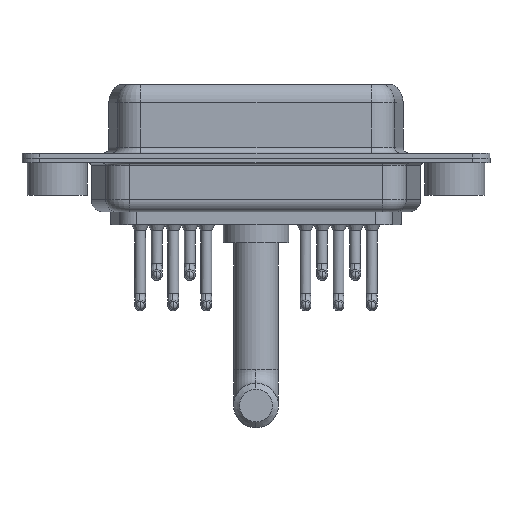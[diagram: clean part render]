
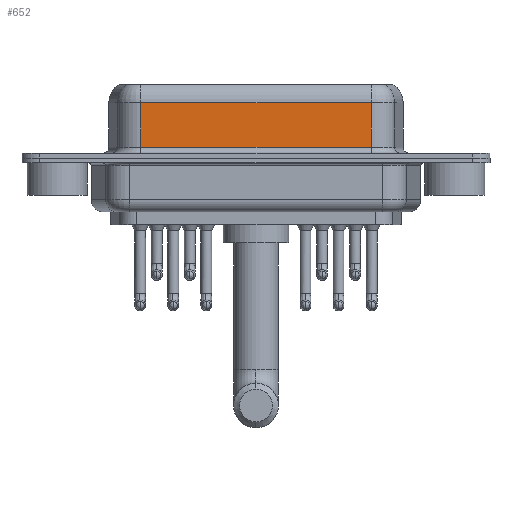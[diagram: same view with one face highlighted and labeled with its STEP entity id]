
A CAD part, front view. The second image highlights one B-rep face of the part: STEP entity #652.
In plain terms, the highlighted planar face has unit normal (0, -1, 0).
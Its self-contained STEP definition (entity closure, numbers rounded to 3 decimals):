
#566 = CARTESIAN_POINT ( 'NONE',  ( 26.287, -3.95, 6.4 ) ) ;
#652 = ADVANCED_FACE ( 'NONE', ( #7935 ), #5292, .F. ) ;
#713 = VERTEX_POINT ( 'NONE', #6616 ) ;
#1874 = VECTOR ( 'NONE', #8198, 1000. ) ;
#2140 = EDGE_CURVE ( 'NONE', #11260, #3890, #15834, .T. ) ;
#2654 = CARTESIAN_POINT ( 'NONE',  ( 26.287, -3.95, 0.9 ) ) ;
#2870 = EDGE_CURVE ( 'NONE', #713, #15268, #16862, .T. ) ;
#3517 = DIRECTION ( 'NONE',  ( 0., 1., 0. ) ) ;
#3848 = ORIENTED_EDGE ( 'NONE', *, *, #12846, .T. ) ;
#3890 = VERTEX_POINT ( 'NONE', #9150 ) ;
#4657 = CARTESIAN_POINT ( 'NONE',  ( 26.287, -3.95, 0.9 ) ) ;
#4735 = DIRECTION ( 'NONE',  ( -1., 0., 0. ) ) ;
#5209 = EDGE_LOOP ( 'NONE', ( #10716, #3848, #16839, #12784 ) ) ;
#5292 = PLANE ( 'NONE',  #7960 ) ;
#5393 = DIRECTION ( 'NONE',  ( 1., 0., 0. ) ) ;
#6616 = CARTESIAN_POINT ( 'NONE',  ( 26.287, -3.95, 4.65 ) ) ;
#6799 = LINE ( 'NONE', #2654, #14232 ) ;
#7274 = LINE ( 'NONE', #8706, #11111 ) ;
#7935 = FACE_OUTER_BOUND ( 'NONE', #5209, .T. ) ;
#7960 = AXIS2_PLACEMENT_3D ( 'NONE', #566, #3517, #13483 ) ;
#8198 = DIRECTION ( 'NONE',  ( 0., 0., -1. ) ) ;
#8706 = CARTESIAN_POINT ( 'NONE',  ( 26.287, -3.95, 4.65 ) ) ;
#9150 = CARTESIAN_POINT ( 'NONE',  ( 7.013, -3.95, 0.9 ) ) ;
#9880 = CARTESIAN_POINT ( 'NONE',  ( 26.287, -3.95, 6.4 ) ) ;
#10716 = ORIENTED_EDGE ( 'NONE', *, *, #2870, .F. ) ;
#11111 = VECTOR ( 'NONE', #4735, 1000. ) ;
#11260 = VERTEX_POINT ( 'NONE', #12091 ) ;
#11391 = CARTESIAN_POINT ( 'NONE',  ( 7.013, -3.95, 6.4 ) ) ;
#12091 = CARTESIAN_POINT ( 'NONE',  ( 7.013, -3.95, 4.65 ) ) ;
#12784 = ORIENTED_EDGE ( 'NONE', *, *, #13166, .T. ) ;
#12846 = EDGE_CURVE ( 'NONE', #713, #11260, #7274, .T. ) ;
#12890 = DIRECTION ( 'NONE',  ( 0., 0., -1. ) ) ;
#13166 = EDGE_CURVE ( 'NONE', #3890, #15268, #6799, .T. ) ;
#13483 = DIRECTION ( 'NONE',  ( 0., 0., 1. ) ) ;
#14232 = VECTOR ( 'NONE', #5393, 1000. ) ;
#15268 = VERTEX_POINT ( 'NONE', #4657 ) ;
#15834 = LINE ( 'NONE', #11391, #16290 ) ;
#16290 = VECTOR ( 'NONE', #12890, 1000. ) ;
#16839 = ORIENTED_EDGE ( 'NONE', *, *, #2140, .T. ) ;
#16862 = LINE ( 'NONE', #9880, #1874 ) ;
